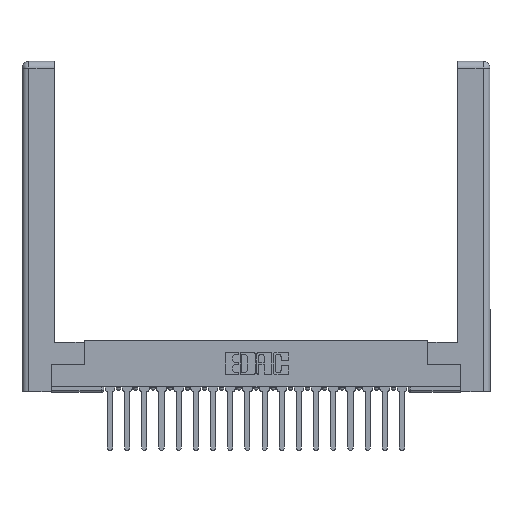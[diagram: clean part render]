
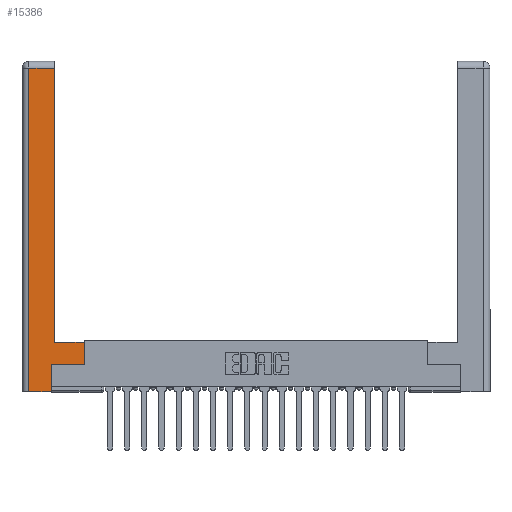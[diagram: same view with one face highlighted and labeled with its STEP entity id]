
A CAD part, top view. The second image highlights one B-rep face of the part: STEP entity #15386.
In plain terms, the highlighted planar face has unit normal (0, 0, 1).
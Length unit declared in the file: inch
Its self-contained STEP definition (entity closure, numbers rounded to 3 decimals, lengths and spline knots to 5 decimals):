
#665 = LINE ( 'NONE', #20085, #19062 ) ;
#1130 = CARTESIAN_POINT ( 'NONE',  ( 0.565, 0.45, 0. ) ) ;
#1586 = PLANE ( 'NONE',  #1874 ) ;
#1874 = AXIS2_PLACEMENT_3D ( 'NONE', #16352, #14534, #16460 ) ;
#2374 = EDGE_CURVE ( 'NONE', #11086, #7266, #10853, .T. ) ;
#2419 = VERTEX_POINT ( 'NONE', #14558 ) ;
#2488 = VERTEX_POINT ( 'NONE', #4589 ) ;
#2491 = LINE ( 'NONE', #15568, #6325 ) ;
#2684 = CARTESIAN_POINT ( 'NONE',  ( 0.565, 0.45, 0. ) ) ;
#2761 = LINE ( 'NONE', #19228, #4263 ) ;
#2989 = DIRECTION ( 'NONE',  ( -1., 0., 0. ) ) ;
#3360 = LINE ( 'NONE', #4956, #10878 ) ;
#3608 = VERTEX_POINT ( 'NONE', #13859 ) ;
#3792 = VERTEX_POINT ( 'NONE', #8201 ) ;
#4263 = VECTOR ( 'NONE', #7659, 39.37008 ) ;
#4585 = CARTESIAN_POINT ( 'NONE',  ( 0.295, 0.45, 0. ) ) ;
#4589 = CARTESIAN_POINT ( 'NONE',  ( 0.265, 0.245, 0. ) ) ;
#4698 = EDGE_CURVE ( 'NONE', #7266, #3792, #9266, .T. ) ;
#4868 = FACE_OUTER_BOUND ( 'NONE', #8254, .T. ) ;
#4956 = CARTESIAN_POINT ( 'NONE',  ( 0.265, 0., 0. ) ) ;
#5383 = CARTESIAN_POINT ( 'NONE',  ( 0.265, 0.245, 0. ) ) ;
#5769 = ORIENTED_EDGE ( 'NONE', *, *, #15313, .T. ) ;
#6090 = DIRECTION ( 'NONE',  ( 0., 1., 0. ) ) ;
#6325 = VECTOR ( 'NONE', #20348, 39.37008 ) ;
#6789 = EDGE_CURVE ( 'NONE', #3608, #13049, #17193, .T. ) ;
#7130 = EDGE_CURVE ( 'NONE', #11737, #2488, #15158, .T. ) ;
#7266 = VERTEX_POINT ( 'NONE', #1130 ) ;
#7545 = CARTESIAN_POINT ( 'NONE',  ( 0.265, 0., 0. ) ) ;
#7659 = DIRECTION ( 'NONE',  ( 0., 1., 0. ) ) ;
#8201 = CARTESIAN_POINT ( 'NONE',  ( 0.295, 0.45, 0. ) ) ;
#8254 = EDGE_LOOP ( 'NONE', ( #5769, #10341, #16259, #14330, #20039, #15626, #10340, #12852 ) ) ;
#8292 = EDGE_CURVE ( 'NONE', #13049, #11737, #3360, .T. ) ;
#8652 = VECTOR ( 'NONE', #6090, 39.37008 ) ;
#9266 = LINE ( 'NONE', #4585, #12693 ) ;
#9423 = DIRECTION ( 'NONE',  ( 0., -1., 0. ) ) ;
#10153 = DIRECTION ( 'NONE',  ( 0., 1., 0. ) ) ;
#10340 = ORIENTED_EDGE ( 'NONE', *, *, #2374, .T. ) ;
#10341 = ORIENTED_EDGE ( 'NONE', *, *, #16172, .T. ) ;
#10853 = LINE ( 'NONE', #2684, #8652 ) ;
#10878 = VECTOR ( 'NONE', #14617, 39.37008 ) ;
#11086 = VERTEX_POINT ( 'NONE', #12985 ) ;
#11737 = VERTEX_POINT ( 'NONE', #7545 ) ;
#11763 = CARTESIAN_POINT ( 'NONE',  ( 0.0615, 0., 0. ) ) ;
#12693 = VECTOR ( 'NONE', #2989, 39.37008 ) ;
#12852 = ORIENTED_EDGE ( 'NONE', *, *, #4698, .T. ) ;
#12985 = CARTESIAN_POINT ( 'NONE',  ( 0.565, 0.245, 0. ) ) ;
#13049 = VERTEX_POINT ( 'NONE', #11763 ) ;
#13798 = DIRECTION ( 'NONE',  ( 1., 0., 0. ) ) ;
#13838 = EDGE_CURVE ( 'NONE', #2488, #11086, #665, .T. ) ;
#13859 = CARTESIAN_POINT ( 'NONE',  ( 0.0615, 2.94, 0. ) ) ;
#14330 = ORIENTED_EDGE ( 'NONE', *, *, #8292, .T. ) ;
#14534 = DIRECTION ( 'NONE',  ( 0., 0., -1. ) ) ;
#14558 = CARTESIAN_POINT ( 'NONE',  ( 0.295, 2.94, 0. ) ) ;
#14617 = DIRECTION ( 'NONE',  ( 1., 0., 0. ) ) ;
#15158 = LINE ( 'NONE', #5383, #18719 ) ;
#15313 = EDGE_CURVE ( 'NONE', #3792, #2419, #2761, .T. ) ;
#15386 = ADVANCED_FACE ( 'NONE', ( #4868 ), #1586, .F. ) ;
#15568 = CARTESIAN_POINT ( 'NONE',  ( 0.0615, 2.94, 0. ) ) ;
#15626 = ORIENTED_EDGE ( 'NONE', *, *, #13838, .T. ) ;
#16006 = CARTESIAN_POINT ( 'NONE',  ( 0.0615, 0., 0. ) ) ;
#16172 = EDGE_CURVE ( 'NONE', #2419, #3608, #2491, .T. ) ;
#16259 = ORIENTED_EDGE ( 'NONE', *, *, #6789, .T. ) ;
#16352 = CARTESIAN_POINT ( 'NONE',  ( 0., 0., 0. ) ) ;
#16460 = DIRECTION ( 'NONE',  ( -1., 0., 0. ) ) ;
#16824 = VECTOR ( 'NONE', #9423, 39.37008 ) ;
#17193 = LINE ( 'NONE', #16006, #16824 ) ;
#18719 = VECTOR ( 'NONE', #10153, 39.37008 ) ;
#19062 = VECTOR ( 'NONE', #13798, 39.37008 ) ;
#19228 = CARTESIAN_POINT ( 'NONE',  ( 0.295, 3., 0. ) ) ;
#20039 = ORIENTED_EDGE ( 'NONE', *, *, #7130, .T. ) ;
#20085 = CARTESIAN_POINT ( 'NONE',  ( 0.565, 0.245, 0. ) ) ;
#20348 = DIRECTION ( 'NONE',  ( -1., 0., 0. ) ) ;
